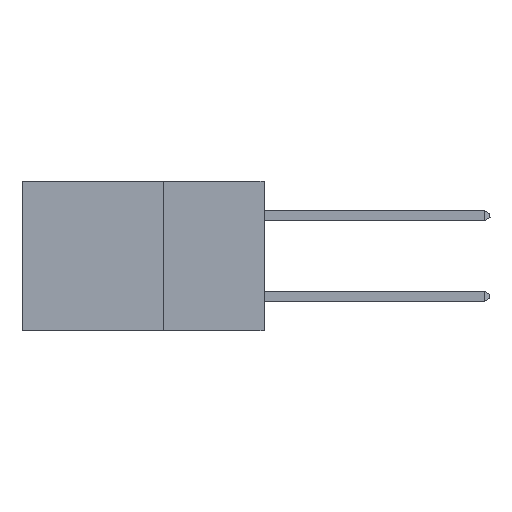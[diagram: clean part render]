
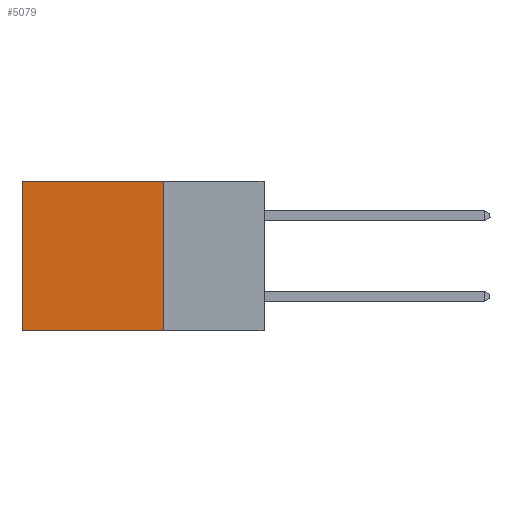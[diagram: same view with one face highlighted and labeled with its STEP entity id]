
A CAD part, left-side view. The second image highlights one B-rep face of the part: STEP entity #5079.
In plain terms, the highlighted planar face has unit normal (-1, 0, 0).
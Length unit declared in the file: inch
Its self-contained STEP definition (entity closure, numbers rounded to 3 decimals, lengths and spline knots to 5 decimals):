
#191 = DIRECTION ( 'NONE',  ( 0., 0., -1. ) ) ;
#1144 = LINE ( 'NONE', #14787, #7318 ) ;
#1581 = LINE ( 'NONE', #3983, #15524 ) ;
#2868 = DIRECTION ( 'NONE',  ( 0., 0., -1. ) ) ;
#3953 = CARTESIAN_POINT ( 'NONE',  ( 0.298, 0.25, 0. ) ) ;
#3983 = CARTESIAN_POINT ( 'NONE',  ( 0.298, 0.25, -0.37 ) ) ;
#5079 = ADVANCED_FACE ( 'NONE', ( #17025 ), #21106, .F. ) ;
#5764 = DIRECTION ( 'NONE',  ( 0., 1., 0. ) ) ;
#5767 = CARTESIAN_POINT ( 'NONE',  ( 0.298, 0.6, 0. ) ) ;
#6173 = VERTEX_POINT ( 'NONE', #12457 ) ;
#6337 = AXIS2_PLACEMENT_3D ( 'NONE', #3953, #9015, #7608 ) ;
#6425 = ORIENTED_EDGE ( 'NONE', *, *, #11299, .F. ) ;
#6578 = ORIENTED_EDGE ( 'NONE', *, *, #13487, .T. ) ;
#7318 = VECTOR ( 'NONE', #2868, 39.37008 ) ;
#7608 = DIRECTION ( 'NONE',  ( 0., 0., -1. ) ) ;
#8306 = DIRECTION ( 'NONE',  ( 0., 1., 0. ) ) ;
#9015 = DIRECTION ( 'NONE',  ( 1., 0., 0. ) ) ;
#9372 = VERTEX_POINT ( 'NONE', #14772 ) ;
#9555 = EDGE_CURVE ( 'NONE', #6173, #9372, #1581, .T. ) ;
#10299 = CARTESIAN_POINT ( 'NONE',  ( 0.298, 0.6, 0. ) ) ;
#11299 = EDGE_CURVE ( 'NONE', #19413, #6173, #1144, .T. ) ;
#11808 = CARTESIAN_POINT ( 'NONE',  ( 0.298, 0.25, 0. ) ) ;
#12457 = CARTESIAN_POINT ( 'NONE',  ( 0.298, 0.25, -0.37 ) ) ;
#13487 = EDGE_CURVE ( 'NONE', #14200, #9372, #19018, .T. ) ;
#13498 = LINE ( 'NONE', #18535, #16699 ) ;
#13556 = ORIENTED_EDGE ( 'NONE', *, *, #15552, .T. ) ;
#14200 = VERTEX_POINT ( 'NONE', #5767 ) ;
#14772 = CARTESIAN_POINT ( 'NONE',  ( 0.298, 0.6, -0.37 ) ) ;
#14787 = CARTESIAN_POINT ( 'NONE',  ( 0.298, 0.25, 0. ) ) ;
#15524 = VECTOR ( 'NONE', #5764, 39.37008 ) ;
#15552 = EDGE_CURVE ( 'NONE', #19413, #14200, #13498, .T. ) ;
#16699 = VECTOR ( 'NONE', #8306, 39.37008 ) ;
#16925 = EDGE_LOOP ( 'NONE', ( #6578, #21782, #6425, #13556 ) ) ;
#17025 = FACE_OUTER_BOUND ( 'NONE', #16925, .T. ) ;
#18535 = CARTESIAN_POINT ( 'NONE',  ( 0.298, 0.25, 0. ) ) ;
#19018 = LINE ( 'NONE', #10299, #21936 ) ;
#19413 = VERTEX_POINT ( 'NONE', #11808 ) ;
#21106 = PLANE ( 'NONE',  #6337 ) ;
#21782 = ORIENTED_EDGE ( 'NONE', *, *, #9555, .F. ) ;
#21936 = VECTOR ( 'NONE', #191, 39.37008 ) ;
